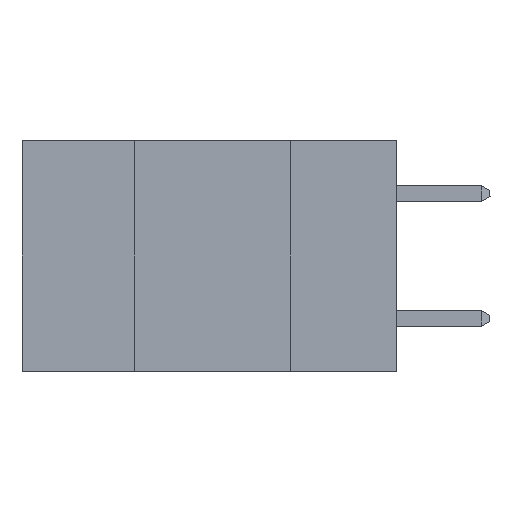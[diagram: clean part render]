
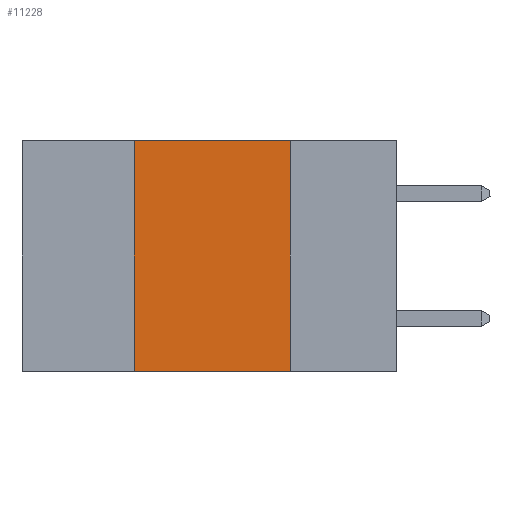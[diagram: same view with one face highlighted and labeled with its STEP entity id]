
A CAD part, left-side view. The second image highlights one B-rep face of the part: STEP entity #11228.
In plain terms, the highlighted planar face has unit normal (-1, 0, 0).
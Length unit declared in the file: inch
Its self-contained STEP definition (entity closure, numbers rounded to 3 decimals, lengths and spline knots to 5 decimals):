
#79 = VERTEX_POINT ( 'NONE', #15276 ) ;
#773 = VERTEX_POINT ( 'NONE', #21193 ) ;
#1831 = LINE ( 'NONE', #26641, #4137 ) ;
#2576 = CARTESIAN_POINT ( 'NONE',  ( 0., 0.6, 0. ) ) ;
#3253 = AXIS2_PLACEMENT_3D ( 'NONE', #15088, #20247, #24753 ) ;
#4137 = VECTOR ( 'NONE', #9580, 39.37008 ) ;
#7081 = VERTEX_POINT ( 'NONE', #20670 ) ;
#7767 = CARTESIAN_POINT ( 'NONE',  ( 0., 0.42, -0.37 ) ) ;
#9580 = DIRECTION ( 'NONE',  ( 0., 0., 1. ) ) ;
#11228 = ADVANCED_FACE ( 'NONE', ( #21055 ), #14982, .F. ) ;
#12382 = DIRECTION ( 'NONE',  ( 0., 0., -1. ) ) ;
#14555 = LINE ( 'NONE', #26157, #20223 ) ;
#14982 = PLANE ( 'NONE',  #3253 ) ;
#15088 = CARTESIAN_POINT ( 'NONE',  ( 0., 0.6, 0. ) ) ;
#15276 = CARTESIAN_POINT ( 'NONE',  ( 0., 0.42, 0. ) ) ;
#16260 = ORIENTED_EDGE ( 'NONE', *, *, #18859, .F. ) ;
#17729 = VERTEX_POINT ( 'NONE', #7767 ) ;
#17896 = VECTOR ( 'NONE', #26484, 39.37008 ) ;
#18859 = EDGE_CURVE ( 'NONE', #17729, #79, #1831, .T. ) ;
#19031 = LINE ( 'NONE', #2576, #17896 ) ;
#20223 = VECTOR ( 'NONE', #30745, 39.37008 ) ;
#20247 = DIRECTION ( 'NONE',  ( 1., 0., 0. ) ) ;
#20670 = CARTESIAN_POINT ( 'NONE',  ( 0., 0.17, 0. ) ) ;
#21055 = FACE_OUTER_BOUND ( 'NONE', #21402, .T. ) ;
#21193 = CARTESIAN_POINT ( 'NONE',  ( 0., 0.17, -0.37 ) ) ;
#21402 = EDGE_LOOP ( 'NONE', ( #27471, #23703, #16260, #23981 ) ) ;
#21907 = CARTESIAN_POINT ( 'NONE',  ( 0., 0.17, 0. ) ) ;
#21983 = EDGE_CURVE ( 'NONE', #79, #7081, #19031, .T. ) ;
#22122 = EDGE_CURVE ( 'NONE', #7081, #773, #27747, .T. ) ;
#23703 = ORIENTED_EDGE ( 'NONE', *, *, #21983, .F. ) ;
#23981 = ORIENTED_EDGE ( 'NONE', *, *, #26344, .T. ) ;
#24753 = DIRECTION ( 'NONE',  ( 0., 0., -1. ) ) ;
#26157 = CARTESIAN_POINT ( 'NONE',  ( 0., 0.6, -0.37 ) ) ;
#26344 = EDGE_CURVE ( 'NONE', #17729, #773, #14555, .T. ) ;
#26484 = DIRECTION ( 'NONE',  ( 0., -1., 0. ) ) ;
#26641 = CARTESIAN_POINT ( 'NONE',  ( 0., 0.42, 0. ) ) ;
#27471 = ORIENTED_EDGE ( 'NONE', *, *, #22122, .F. ) ;
#27747 = LINE ( 'NONE', #21907, #29616 ) ;
#29616 = VECTOR ( 'NONE', #12382, 39.37008 ) ;
#30745 = DIRECTION ( 'NONE',  ( 0., -1., 0. ) ) ;
